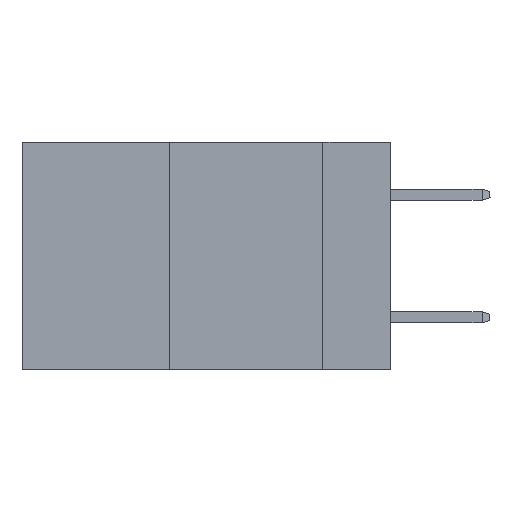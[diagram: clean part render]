
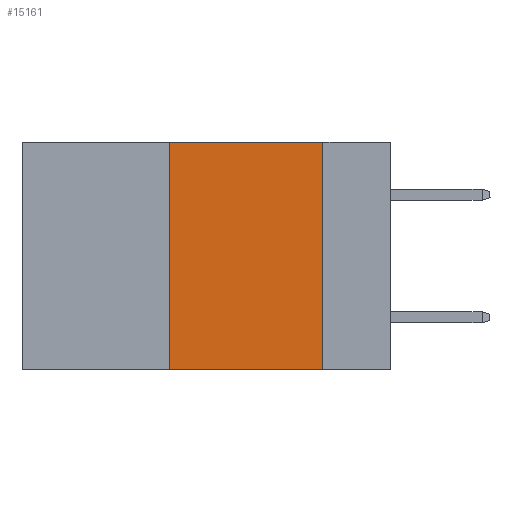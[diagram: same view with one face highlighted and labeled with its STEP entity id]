
A CAD part, left-side view. The second image highlights one B-rep face of the part: STEP entity #15161.
In plain terms, the highlighted planar face has unit normal (-1, 0, 0).
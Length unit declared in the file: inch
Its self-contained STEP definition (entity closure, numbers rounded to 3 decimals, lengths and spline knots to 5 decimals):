
#316 = ORIENTED_EDGE ( 'NONE', *, *, #2824, .F. ) ;
#380 = VERTEX_POINT ( 'NONE', #4185 ) ;
#1529 = LINE ( 'NONE', #3254, #8775 ) ;
#2057 = FACE_OUTER_BOUND ( 'NONE', #2894, .T. ) ;
#2133 = DIRECTION ( 'NONE',  ( 0., 0., -1. ) ) ;
#2243 = DIRECTION ( 'NONE',  ( 0., -1., 0. ) ) ;
#2722 = EDGE_CURVE ( 'NONE', #9869, #4836, #16094, .T. ) ;
#2824 = EDGE_CURVE ( 'NONE', #380, #11184, #8479, .T. ) ;
#2894 = EDGE_LOOP ( 'NONE', ( #316, #7773, #7092, #12709 ) ) ;
#3117 = CARTESIAN_POINT ( 'NONE',  ( 0., 0.36, 0. ) ) ;
#3254 = CARTESIAN_POINT ( 'NONE',  ( 0., 0.6, -0.37 ) ) ;
#4094 = CARTESIAN_POINT ( 'NONE',  ( 0., 0.36, -0.37 ) ) ;
#4185 = CARTESIAN_POINT ( 'NONE',  ( 0., 0.11, 0. ) ) ;
#4341 = DIRECTION ( 'NONE',  ( 0., -1., 0. ) ) ;
#4836 = VERTEX_POINT ( 'NONE', #8191 ) ;
#4969 = DIRECTION ( 'NONE',  ( 1., 0., 0. ) ) ;
#5466 = EDGE_CURVE ( 'NONE', #9869, #11184, #1529, .T. ) ;
#6061 = LINE ( 'NONE', #14864, #10921 ) ;
#6206 = CARTESIAN_POINT ( 'NONE',  ( 0., 0.6, 0. ) ) ;
#6836 = DIRECTION ( 'NONE',  ( 0., 0., 1. ) ) ;
#6991 = CARTESIAN_POINT ( 'NONE',  ( 0., 0.11, 0. ) ) ;
#7092 = ORIENTED_EDGE ( 'NONE', *, *, #2722, .F. ) ;
#7400 = PLANE ( 'NONE',  #11043 ) ;
#7773 = ORIENTED_EDGE ( 'NONE', *, *, #13081, .F. ) ;
#8191 = CARTESIAN_POINT ( 'NONE',  ( 0., 0.36, 0. ) ) ;
#8479 = LINE ( 'NONE', #6991, #12779 ) ;
#8775 = VECTOR ( 'NONE', #2243, 39.37008 ) ;
#9435 = VECTOR ( 'NONE', #6836, 39.37008 ) ;
#9869 = VERTEX_POINT ( 'NONE', #4094 ) ;
#10921 = VECTOR ( 'NONE', #4341, 39.37008 ) ;
#11043 = AXIS2_PLACEMENT_3D ( 'NONE', #6206, #4969, #13729 ) ;
#11184 = VERTEX_POINT ( 'NONE', #15764 ) ;
#12709 = ORIENTED_EDGE ( 'NONE', *, *, #5466, .T. ) ;
#12779 = VECTOR ( 'NONE', #2133, 39.37008 ) ;
#13081 = EDGE_CURVE ( 'NONE', #4836, #380, #6061, .T. ) ;
#13729 = DIRECTION ( 'NONE',  ( 0., 0., -1. ) ) ;
#14864 = CARTESIAN_POINT ( 'NONE',  ( 0., 0.6, 0. ) ) ;
#15161 = ADVANCED_FACE ( 'NONE', ( #2057 ), #7400, .F. ) ;
#15764 = CARTESIAN_POINT ( 'NONE',  ( 0., 0.11, -0.37 ) ) ;
#16094 = LINE ( 'NONE', #3117, #9435 ) ;
